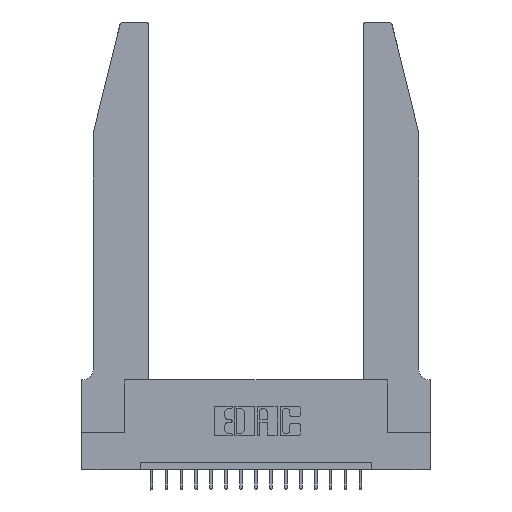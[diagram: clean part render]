
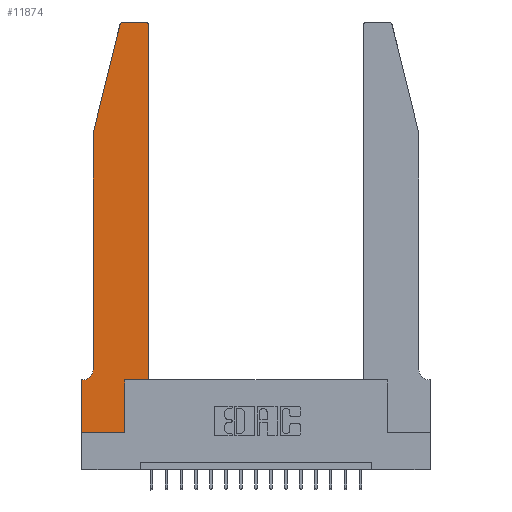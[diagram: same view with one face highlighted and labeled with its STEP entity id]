
A CAD part, top view. The second image highlights one B-rep face of the part: STEP entity #11874.
In plain terms, the highlighted planar face has unit normal (0, 0, 1).
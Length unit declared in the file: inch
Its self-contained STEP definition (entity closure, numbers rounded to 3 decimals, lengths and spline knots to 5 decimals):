
#191 = EDGE_CURVE ( 'NONE', #14547, #16496, #18774, .T. ) ;
#310 = VERTEX_POINT ( 'NONE', #15870 ) ;
#327 = VERTEX_POINT ( 'NONE', #10097 ) ;
#350 = VECTOR ( 'NONE', #9372, 39.37008 ) ;
#509 = DIRECTION ( 'NONE',  ( 1., 0., 0. ) ) ;
#1468 = DIRECTION ( 'NONE',  ( 0., 0., -1. ) ) ;
#1736 = CARTESIAN_POINT ( 'NONE',  ( 0.0755, 2., 0.37 ) ) ;
#1812 = LINE ( 'NONE', #10590, #6996 ) ;
#1970 = AXIS2_PLACEMENT_3D ( 'NONE', #6236, #1468, #9260 ) ;
#2015 = FACE_OUTER_BOUND ( 'NONE', #2488, .T. ) ;
#2312 = CARTESIAN_POINT ( 'NONE',  ( 0.284, 2.75, 0.37 ) ) ;
#2488 = EDGE_LOOP ( 'NONE', ( #10376, #17149, #8641, #5407, #3635, #15267, #8183, #17300, #3952, #7475, #6565, #9902 ) ) ;
#2766 = CARTESIAN_POINT ( 'NONE',  ( 0.2865, 0.35, 0.37 ) ) ;
#2976 = LINE ( 'NONE', #15256, #19108 ) ;
#3063 = DIRECTION ( 'NONE',  ( 0., -1., 0. ) ) ;
#3155 = DIRECTION ( 'NONE',  ( -1., 0., 0. ) ) ;
#3336 = EDGE_CURVE ( 'NONE', #16496, #310, #17738, .T. ) ;
#3635 = ORIENTED_EDGE ( 'NONE', *, *, #18384, .T. ) ;
#3952 = ORIENTED_EDGE ( 'NONE', *, *, #14947, .T. ) ;
#4116 = LINE ( 'NONE', #10061, #9892 ) ;
#4366 = CARTESIAN_POINT ( 'NONE',  ( 0.4205, 2.72, 0.37 ) ) ;
#4633 = CARTESIAN_POINT ( 'NONE',  ( 0.0755, 0.35, 0.37 ) ) ;
#4946 = AXIS2_PLACEMENT_3D ( 'NONE', #5027, #8041, #14540 ) ;
#5027 = CARTESIAN_POINT ( 'NONE',  ( 0.284, 2.72, 0.37 ) ) ;
#5080 = CARTESIAN_POINT ( 'NONE',  ( 0.0055, 0.35, 0.37 ) ) ;
#5282 = CARTESIAN_POINT ( 'NONE',  ( 0., 0.35, 0.37 ) ) ;
#5404 = DIRECTION ( 'NONE',  ( 0., 1., 0. ) ) ;
#5407 = ORIENTED_EDGE ( 'NONE', *, *, #11279, .T. ) ;
#5676 = CIRCLE ( 'NONE', #9200, 0.03 ) ;
#5919 = CARTESIAN_POINT ( 'NONE',  ( 0., 0.35, 0.37 ) ) ;
#6236 = CARTESIAN_POINT ( 'NONE',  ( 0.0055, 0.42, 0.37 ) ) ;
#6565 = ORIENTED_EDGE ( 'NONE', *, *, #15375, .T. ) ;
#6996 = VECTOR ( 'NONE', #10504, 39.37008 ) ;
#7336 = VECTOR ( 'NONE', #3063, 39.37008 ) ;
#7360 = VECTOR ( 'NONE', #3155, 39.37008 ) ;
#7475 = ORIENTED_EDGE ( 'NONE', *, *, #19628, .T. ) ;
#7516 = DIRECTION ( 'NONE',  ( 0., -1., 0. ) ) ;
#8041 = DIRECTION ( 'NONE',  ( 0., 0., 1. ) ) ;
#8183 = ORIENTED_EDGE ( 'NONE', *, *, #9149, .T. ) ;
#8318 = VERTEX_POINT ( 'NONE', #18127 ) ;
#8641 = ORIENTED_EDGE ( 'NONE', *, *, #16369, .T. ) ;
#8648 = VECTOR ( 'NONE', #16763, 39.37008 ) ;
#8964 = CARTESIAN_POINT ( 'NONE',  ( 0., 0., 0.37 ) ) ;
#9036 = CARTESIAN_POINT ( 'NONE',  ( 0.0755, 2., 0.37 ) ) ;
#9149 = EDGE_CURVE ( 'NONE', #17545, #12535, #16866, .T. ) ;
#9200 = AXIS2_PLACEMENT_3D ( 'NONE', #4366, #14970, #16393 ) ;
#9260 = DIRECTION ( 'NONE',  ( -1., 0., 0. ) ) ;
#9372 = DIRECTION ( 'NONE',  ( -1., 0., 0. ) ) ;
#9551 = VERTEX_POINT ( 'NONE', #1736 ) ;
#9892 = VECTOR ( 'NONE', #5404, 39.37008 ) ;
#9902 = ORIENTED_EDGE ( 'NONE', *, *, #14731, .T. ) ;
#9920 = PLANE ( 'NONE',  #15808 ) ;
#10061 = CARTESIAN_POINT ( 'NONE',  ( 0.4505, 0.35, 0.37 ) ) ;
#10097 = CARTESIAN_POINT ( 'NONE',  ( 0.2865, 0., 0.37 ) ) ;
#10222 = VERTEX_POINT ( 'NONE', #12279 ) ;
#10376 = ORIENTED_EDGE ( 'NONE', *, *, #191, .T. ) ;
#10504 = DIRECTION ( 'NONE',  ( -0.239, -0.971, 0. ) ) ;
#10575 = DIRECTION ( 'NONE',  ( 1., 0., 0. ) ) ;
#10590 = CARTESIAN_POINT ( 'NONE',  ( 0.0755, 2., 0.37 ) ) ;
#11279 = EDGE_CURVE ( 'NONE', #9551, #8318, #15125, .T. ) ;
#11404 = DIRECTION ( 'NONE',  ( 0., 0., 1. ) ) ;
#11874 = ADVANCED_FACE ( 'NONE', ( #2015 ), #9920, .T. ) ;
#12023 = VERTEX_POINT ( 'NONE', #14736 ) ;
#12057 = LINE ( 'NONE', #4633, #7360 ) ;
#12279 = CARTESIAN_POINT ( 'NONE',  ( 0.4505, 2.72, 0.37 ) ) ;
#12287 = CARTESIAN_POINT ( 'NONE',  ( 0.4205, 2.75, 0.37 ) ) ;
#12535 = VERTEX_POINT ( 'NONE', #16226 ) ;
#12566 = VECTOR ( 'NONE', #7516, 39.37008 ) ;
#13361 = LINE ( 'NONE', #15175, #15376 ) ;
#13436 = LINE ( 'NONE', #19545, #8648 ) ;
#13640 = DIRECTION ( 'NONE',  ( 0., 1., 0. ) ) ;
#14540 = DIRECTION ( 'NONE',  ( 1., 0., 0. ) ) ;
#14547 = VERTEX_POINT ( 'NONE', #12287 ) ;
#14731 = EDGE_CURVE ( 'NONE', #10222, #14547, #5676, .T. ) ;
#14736 = CARTESIAN_POINT ( 'NONE',  ( 0.4505, 0.35, 0.37 ) ) ;
#14947 = EDGE_CURVE ( 'NONE', #327, #17054, #2976, .T. ) ;
#14970 = DIRECTION ( 'NONE',  ( 0., 0., 1. ) ) ;
#15125 = LINE ( 'NONE', #9036, #12566 ) ;
#15175 = CARTESIAN_POINT ( 'NONE',  ( 0.4505, 0.35, 0.37 ) ) ;
#15256 = CARTESIAN_POINT ( 'NONE',  ( 0.2865, 0.35, 0.37 ) ) ;
#15267 = ORIENTED_EDGE ( 'NONE', *, *, #18400, .T. ) ;
#15375 = EDGE_CURVE ( 'NONE', #12023, #10222, #4116, .T. ) ;
#15376 = VECTOR ( 'NONE', #10575, 39.37008 ) ;
#15808 = AXIS2_PLACEMENT_3D ( 'NONE', #5282, #11404, #509 ) ;
#15870 = CARTESIAN_POINT ( 'NONE',  ( 0.25487, 2.72718, 0.37 ) ) ;
#16009 = CIRCLE ( 'NONE', #1970, 0.07 ) ;
#16226 = CARTESIAN_POINT ( 'NONE',  ( 0., 0., 0.37 ) ) ;
#16369 = EDGE_CURVE ( 'NONE', #310, #9551, #1812, .T. ) ;
#16393 = DIRECTION ( 'NONE',  ( 1., 0., 0. ) ) ;
#16496 = VERTEX_POINT ( 'NONE', #2312 ) ;
#16763 = DIRECTION ( 'NONE',  ( 1., 0., 0. ) ) ;
#16866 = LINE ( 'NONE', #8964, #7336 ) ;
#16872 = CARTESIAN_POINT ( 'NONE',  ( 0.2605, 2.75, 0.37 ) ) ;
#17054 = VERTEX_POINT ( 'NONE', #2766 ) ;
#17149 = ORIENTED_EDGE ( 'NONE', *, *, #3336, .T. ) ;
#17300 = ORIENTED_EDGE ( 'NONE', *, *, #18423, .T. ) ;
#17545 = VERTEX_POINT ( 'NONE', #5919 ) ;
#17738 = CIRCLE ( 'NONE', #4946, 0.03 ) ;
#18127 = CARTESIAN_POINT ( 'NONE',  ( 0.0755, 0.42, 0.37 ) ) ;
#18384 = EDGE_CURVE ( 'NONE', #8318, #19324, #16009, .T. ) ;
#18400 = EDGE_CURVE ( 'NONE', #19324, #17545, #12057, .T. ) ;
#18423 = EDGE_CURVE ( 'NONE', #12535, #327, #13436, .T. ) ;
#18774 = LINE ( 'NONE', #16872, #350 ) ;
#19108 = VECTOR ( 'NONE', #13640, 39.37008 ) ;
#19324 = VERTEX_POINT ( 'NONE', #5080 ) ;
#19545 = CARTESIAN_POINT ( 'NONE',  ( 0., 0., 0.37 ) ) ;
#19628 = EDGE_CURVE ( 'NONE', #17054, #12023, #13361, .T. ) ;
